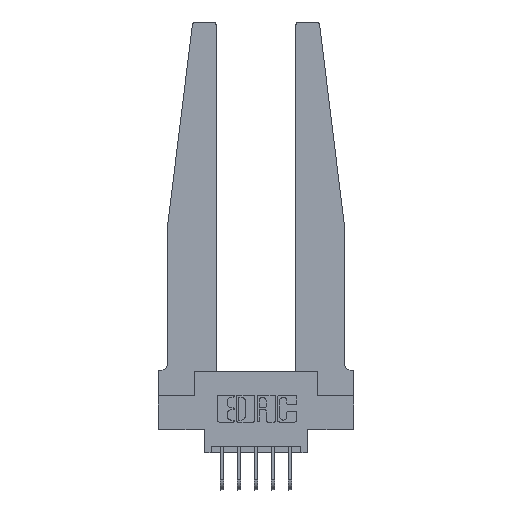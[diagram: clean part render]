
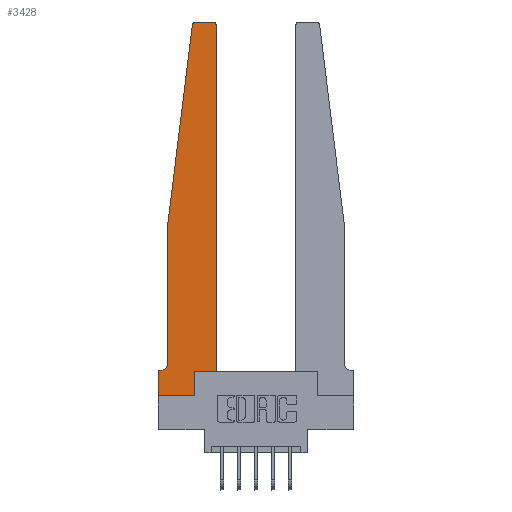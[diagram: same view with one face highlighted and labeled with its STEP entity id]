
A CAD part, top view. The second image highlights one B-rep face of the part: STEP entity #3428.
In plain terms, the highlighted planar face has unit normal (0, 0, 1).
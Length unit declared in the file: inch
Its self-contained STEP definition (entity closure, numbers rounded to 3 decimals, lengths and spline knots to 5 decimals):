
#115 = DIRECTION ( 'NONE',  ( 0., 0., 1. ) ) ;
#164 = CARTESIAN_POINT ( 'NONE',  ( 0.015, 0.1875, 0.37 ) ) ;
#167 = CARTESIAN_POINT ( 'NONE',  ( 0.2605, 0., 0.37 ) ) ;
#352 = DIRECTION ( 'NONE',  ( 1., 0., 0. ) ) ;
#401 = CARTESIAN_POINT ( 'NONE',  ( 0.425, 0.18, 0.37 ) ) ;
#529 = EDGE_CURVE ( 'NONE', #9917, #651, #1450, .T. ) ;
#651 = VERTEX_POINT ( 'NONE', #1231 ) ;
#860 = LINE ( 'NONE', #2084, #1038 ) ;
#1018 = CARTESIAN_POINT ( 'NONE',  ( 0.25, 2.75, 0.37 ) ) ;
#1028 = DIRECTION ( 'NONE',  ( 0., -1., 0. ) ) ;
#1038 = VECTOR ( 'NONE', #12568, 39.37008 ) ;
#1058 = CARTESIAN_POINT ( 'NONE',  ( 0., 0., 0.37 ) ) ;
#1231 = CARTESIAN_POINT ( 'NONE',  ( 0.425, 2.72, 0.37 ) ) ;
#1327 = ORIENTED_EDGE ( 'NONE', *, *, #7982, .T. ) ;
#1450 = LINE ( 'NONE', #401, #1956 ) ;
#1553 = VERTEX_POINT ( 'NONE', #3611 ) ;
#1765 = VERTEX_POINT ( 'NONE', #1058 ) ;
#1956 = VECTOR ( 'NONE', #8728, 39.37008 ) ;
#1986 = LINE ( 'NONE', #4426, #12234 ) ;
#2084 = CARTESIAN_POINT ( 'NONE',  ( 0.2605, 0.18, 0.37 ) ) ;
#2258 = VECTOR ( 'NONE', #7237, 39.37008 ) ;
#2376 = DIRECTION ( 'NONE',  ( 0., 0., 1. ) ) ;
#2400 = EDGE_CURVE ( 'NONE', #1765, #12962, #10322, .T. ) ;
#2425 = ORIENTED_EDGE ( 'NONE', *, *, #6007, .T. ) ;
#2440 = ORIENTED_EDGE ( 'NONE', *, *, #12601, .T. ) ;
#2475 = EDGE_CURVE ( 'NONE', #1553, #9917, #11643, .T. ) ;
#2555 = CARTESIAN_POINT ( 'NONE',  ( 0., 0.1875, 0.37 ) ) ;
#2726 = VERTEX_POINT ( 'NONE', #5643 ) ;
#2873 = VECTOR ( 'NONE', #12676, 39.37008 ) ;
#3109 = LINE ( 'NONE', #12598, #2258 ) ;
#3129 = VERTEX_POINT ( 'NONE', #5528 ) ;
#3268 = DIRECTION ( 'NONE',  ( 1., 0., 0. ) ) ;
#3291 = VECTOR ( 'NONE', #5262, 39.37008 ) ;
#3428 = ADVANCED_FACE ( 'NONE', ( #5393 ), #8544, .T. ) ;
#3611 = CARTESIAN_POINT ( 'NONE',  ( 0.2605, 0.18, 0.37 ) ) ;
#3920 = CARTESIAN_POINT ( 'NONE',  ( 0.24675, 2.72367, 0.37 ) ) ;
#3971 = CARTESIAN_POINT ( 'NONE',  ( 0.065, 1.25, 0.37 ) ) ;
#4094 = LINE ( 'NONE', #1018, #12355 ) ;
#4175 = VECTOR ( 'NONE', #6630, 39.37008 ) ;
#4376 = CARTESIAN_POINT ( 'NONE',  ( 0.425, 0.18, 0.37 ) ) ;
#4426 = CARTESIAN_POINT ( 'NONE',  ( 0.065, 0.1875, 0.37 ) ) ;
#4709 = EDGE_LOOP ( 'NONE', ( #1327, #8034, #2425, #5508, #10127, #2440, #11819, #9875, #6249, #12421, #13490, #9944 ) ) ;
#4860 = AXIS2_PLACEMENT_3D ( 'NONE', #2555, #5459, #352 ) ;
#5206 = LINE ( 'NONE', #9291, #2873 ) ;
#5262 = DIRECTION ( 'NONE',  ( 1., 0., 0. ) ) ;
#5393 = FACE_OUTER_BOUND ( 'NONE', #4709, .T. ) ;
#5459 = DIRECTION ( 'NONE',  ( 0., 0., 1. ) ) ;
#5508 = ORIENTED_EDGE ( 'NONE', *, *, #10397, .T. ) ;
#5517 = EDGE_CURVE ( 'NONE', #9991, #8424, #12965, .T. ) ;
#5528 = CARTESIAN_POINT ( 'NONE',  ( 0.395, 2.75, 0.37 ) ) ;
#5643 = CARTESIAN_POINT ( 'NONE',  ( 0.065, 0.2375, 0.37 ) ) ;
#5745 = CARTESIAN_POINT ( 'NONE',  ( 0.015, 0.2375, 0.37 ) ) ;
#5752 = AXIS2_PLACEMENT_3D ( 'NONE', #8446, #2376, #12766 ) ;
#5817 = DIRECTION ( 'NONE',  ( 0., 0., -1. ) ) ;
#6007 = EDGE_CURVE ( 'NONE', #8424, #6770, #3109, .T. ) ;
#6046 = VECTOR ( 'NONE', #1028, 39.37008 ) ;
#6075 = DIRECTION ( 'NONE',  ( -1., 0., 0. ) ) ;
#6081 = CARTESIAN_POINT ( 'NONE',  ( 0., 0., 0.37 ) ) ;
#6249 = ORIENTED_EDGE ( 'NONE', *, *, #7137, .T. ) ;
#6630 = DIRECTION ( 'NONE',  ( 1., 0., 0. ) ) ;
#6714 = CARTESIAN_POINT ( 'NONE',  ( 0., 0.1875, 0.37 ) ) ;
#6770 = VERTEX_POINT ( 'NONE', #13135 ) ;
#7137 = EDGE_CURVE ( 'NONE', #12962, #1553, #860, .T. ) ;
#7237 = DIRECTION ( 'NONE',  ( -0.122, -0.992, 0. ) ) ;
#7383 = CIRCLE ( 'NONE', #9132, 0.05 ) ;
#7601 = CARTESIAN_POINT ( 'NONE',  ( 0.27653, 2.72, 0.37 ) ) ;
#7982 = EDGE_CURVE ( 'NONE', #3129, #9991, #4094, .T. ) ;
#8034 = ORIENTED_EDGE ( 'NONE', *, *, #5517, .T. ) ;
#8233 = DIRECTION ( 'NONE',  ( -1., 0., 0. ) ) ;
#8424 = VERTEX_POINT ( 'NONE', #3920 ) ;
#8446 = CARTESIAN_POINT ( 'NONE',  ( 0.395, 2.72, 0.37 ) ) ;
#8544 = PLANE ( 'NONE',  #4860 ) ;
#8728 = DIRECTION ( 'NONE',  ( 0., 1., 0. ) ) ;
#9073 = EDGE_CURVE ( 'NONE', #651, #3129, #11889, .T. ) ;
#9128 = CARTESIAN_POINT ( 'NONE',  ( 0.425, 0.18, 0.37 ) ) ;
#9132 = AXIS2_PLACEMENT_3D ( 'NONE', #5745, #5817, #9989 ) ;
#9291 = CARTESIAN_POINT ( 'NONE',  ( 0., 0., 0.37 ) ) ;
#9875 = ORIENTED_EDGE ( 'NONE', *, *, #2400, .T. ) ;
#9917 = VERTEX_POINT ( 'NONE', #9128 ) ;
#9944 = ORIENTED_EDGE ( 'NONE', *, *, #9073, .T. ) ;
#9989 = DIRECTION ( 'NONE',  ( -1., 0., 0. ) ) ;
#9991 = VERTEX_POINT ( 'NONE', #12919 ) ;
#10127 = ORIENTED_EDGE ( 'NONE', *, *, #12256, .T. ) ;
#10322 = LINE ( 'NONE', #6081, #3291 ) ;
#10397 = EDGE_CURVE ( 'NONE', #6770, #2726, #10520, .T. ) ;
#10520 = LINE ( 'NONE', #3971, #6046 ) ;
#11329 = VERTEX_POINT ( 'NONE', #6714 ) ;
#11643 = LINE ( 'NONE', #4376, #4175 ) ;
#11819 = ORIENTED_EDGE ( 'NONE', *, *, #13361, .T. ) ;
#11889 = CIRCLE ( 'NONE', #5752, 0.03 ) ;
#11986 = VERTEX_POINT ( 'NONE', #164 ) ;
#12234 = VECTOR ( 'NONE', #6075, 39.37008 ) ;
#12256 = EDGE_CURVE ( 'NONE', #2726, #11986, #7383, .T. ) ;
#12297 = AXIS2_PLACEMENT_3D ( 'NONE', #7601, #115, #3268 ) ;
#12355 = VECTOR ( 'NONE', #8233, 39.37008 ) ;
#12421 = ORIENTED_EDGE ( 'NONE', *, *, #2475, .T. ) ;
#12568 = DIRECTION ( 'NONE',  ( 0., 1., 0. ) ) ;
#12598 = CARTESIAN_POINT ( 'NONE',  ( 0.065, 1.25, 0.37 ) ) ;
#12601 = EDGE_CURVE ( 'NONE', #11986, #11329, #1986, .T. ) ;
#12676 = DIRECTION ( 'NONE',  ( 0., -1., 0. ) ) ;
#12766 = DIRECTION ( 'NONE',  ( 1., 0., 0. ) ) ;
#12919 = CARTESIAN_POINT ( 'NONE',  ( 0.27653, 2.75, 0.37 ) ) ;
#12962 = VERTEX_POINT ( 'NONE', #167 ) ;
#12965 = CIRCLE ( 'NONE', #12297, 0.03 ) ;
#13135 = CARTESIAN_POINT ( 'NONE',  ( 0.065, 1.25, 0.37 ) ) ;
#13361 = EDGE_CURVE ( 'NONE', #11329, #1765, #5206, .T. ) ;
#13490 = ORIENTED_EDGE ( 'NONE', *, *, #529, .T. ) ;
